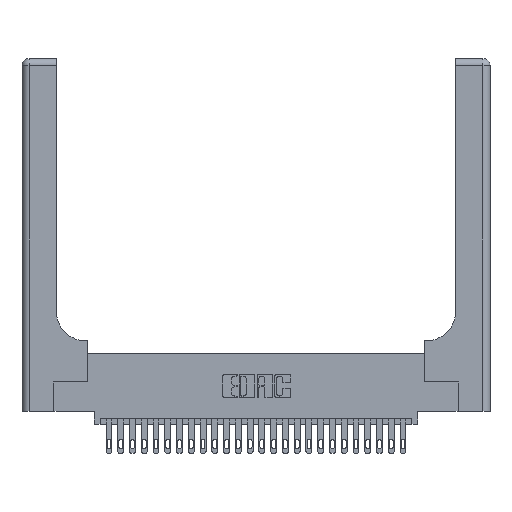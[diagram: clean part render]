
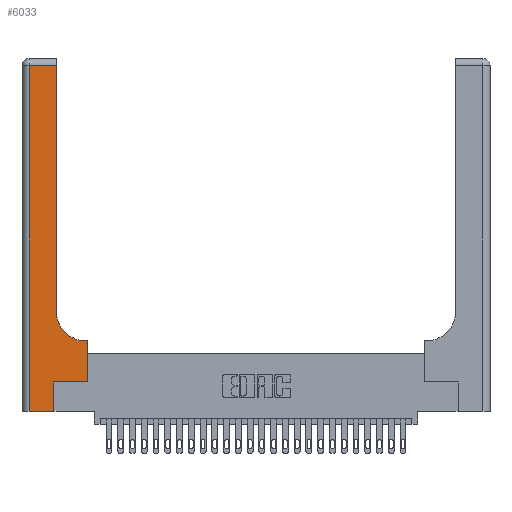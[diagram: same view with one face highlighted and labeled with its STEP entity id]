
A CAD part, top view. The second image highlights one B-rep face of the part: STEP entity #6033.
In plain terms, the highlighted planar face has unit normal (0, 0, 1).
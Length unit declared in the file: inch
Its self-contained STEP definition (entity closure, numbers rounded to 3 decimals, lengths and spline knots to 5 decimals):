
#131 = DIRECTION ( 'NONE',  ( 0., 0., -1. ) ) ;
#439 = LINE ( 'NONE', #20734, #23279 ) ;
#657 = CARTESIAN_POINT ( 'NONE',  ( 0., 2.94, 0.37 ) ) ;
#1019 = CARTESIAN_POINT ( 'NONE',  ( 0.269, 0.25, 0.37 ) ) ;
#2223 = ORIENTED_EDGE ( 'NONE', *, *, #15718, .T. ) ;
#2623 = ORIENTED_EDGE ( 'NONE', *, *, #4432, .T. ) ;
#2744 = VECTOR ( 'NONE', #12373, 39.37008 ) ;
#3171 = CARTESIAN_POINT ( 'NONE',  ( 0.269, 0.25, 0.37 ) ) ;
#3258 = VERTEX_POINT ( 'NONE', #15437 ) ;
#3762 = VERTEX_POINT ( 'NONE', #20997 ) ;
#3806 = CARTESIAN_POINT ( 'NONE',  ( 0.5585, 0.25, 0.37 ) ) ;
#3912 = VECTOR ( 'NONE', #10980, 39.37008 ) ;
#4432 = EDGE_CURVE ( 'NONE', #26588, #23386, #439, .T. ) ;
#4525 = CARTESIAN_POINT ( 'NONE',  ( 0., 3., 0.37 ) ) ;
#4573 = CARTESIAN_POINT ( 'NONE',  ( 0.2915, 0.6, 0.37 ) ) ;
#4700 = CARTESIAN_POINT ( 'NONE',  ( 0.269, 0., 0.37 ) ) ;
#5062 = VERTEX_POINT ( 'NONE', #1019 ) ;
#5669 = EDGE_CURVE ( 'NONE', #23386, #22451, #6410, .T. ) ;
#6033 = ADVANCED_FACE ( 'NONE', ( #26609 ), #24020, .F. ) ;
#6235 = CIRCLE ( 'NONE', #26925, 0.25 ) ;
#6410 = LINE ( 'NONE', #657, #2744 ) ;
#6524 = CARTESIAN_POINT ( 'NONE',  ( 0.5415, 0.85, 0.37 ) ) ;
#6826 = DIRECTION ( 'NONE',  ( 0., 1., 0. ) ) ;
#7427 = EDGE_LOOP ( 'NONE', ( #2623, #25507, #14229, #8753, #17224, #18678, #21669, #18323, #2223 ) ) ;
#8072 = EDGE_CURVE ( 'NONE', #3762, #5062, #15392, .T. ) ;
#8261 = LINE ( 'NONE', #8985, #3912 ) ;
#8492 = VERTEX_POINT ( 'NONE', #23797 ) ;
#8753 = ORIENTED_EDGE ( 'NONE', *, *, #17259, .T. ) ;
#8958 = CARTESIAN_POINT ( 'NONE',  ( 0.2915, 0.85, 0.37 ) ) ;
#8985 = CARTESIAN_POINT ( 'NONE',  ( 0.06, 3., 0.37 ) ) ;
#9343 = CARTESIAN_POINT ( 'NONE',  ( 0.2915, 2.94, 0.37 ) ) ;
#9807 = EDGE_CURVE ( 'NONE', #22451, #3258, #8261, .T. ) ;
#10113 = DIRECTION ( 'NONE',  ( 0., 1., 0. ) ) ;
#10292 = LINE ( 'NONE', #4573, #13983 ) ;
#10453 = VECTOR ( 'NONE', #11861, 39.37008 ) ;
#10499 = EDGE_CURVE ( 'NONE', #8492, #21233, #10292, .T. ) ;
#10980 = DIRECTION ( 'NONE',  ( 0., -1., 0. ) ) ;
#11861 = DIRECTION ( 'NONE',  ( 0., 1., 0. ) ) ;
#12165 = LINE ( 'NONE', #27069, #27005 ) ;
#12373 = DIRECTION ( 'NONE',  ( -1., 0., 0. ) ) ;
#12579 = VERTEX_POINT ( 'NONE', #23634 ) ;
#13983 = VECTOR ( 'NONE', #24171, 39.37008 ) ;
#14229 = ORIENTED_EDGE ( 'NONE', *, *, #9807, .T. ) ;
#14825 = LINE ( 'NONE', #3806, #10453 ) ;
#15392 = LINE ( 'NONE', #4700, #23783 ) ;
#15437 = CARTESIAN_POINT ( 'NONE',  ( 0.06, 0., 0.37 ) ) ;
#15718 = EDGE_CURVE ( 'NONE', #21233, #26588, #6235, .T. ) ;
#16834 = DIRECTION ( 'NONE',  ( 1., 0., 0. ) ) ;
#17222 = CARTESIAN_POINT ( 'NONE',  ( 0.5415, 0.6, 0.37 ) ) ;
#17224 = ORIENTED_EDGE ( 'NONE', *, *, #8072, .T. ) ;
#17259 = EDGE_CURVE ( 'NONE', #3258, #3762, #12165, .T. ) ;
#18179 = DIRECTION ( 'NONE',  ( 1., 0., 0. ) ) ;
#18323 = ORIENTED_EDGE ( 'NONE', *, *, #10499, .T. ) ;
#18451 = EDGE_CURVE ( 'NONE', #12579, #8492, #14825, .T. ) ;
#18678 = ORIENTED_EDGE ( 'NONE', *, *, #23442, .T. ) ;
#19542 = DIRECTION ( 'NONE',  ( -1., 0., 0. ) ) ;
#20734 = CARTESIAN_POINT ( 'NONE',  ( 0.2915, 3., 0.37 ) ) ;
#20775 = CARTESIAN_POINT ( 'NONE',  ( 0.06, 2.94, 0.37 ) ) ;
#20827 = VECTOR ( 'NONE', #18179, 39.37008 ) ;
#20997 = CARTESIAN_POINT ( 'NONE',  ( 0.269, 0., 0.37 ) ) ;
#21233 = VERTEX_POINT ( 'NONE', #17222 ) ;
#21669 = ORIENTED_EDGE ( 'NONE', *, *, #18451, .T. ) ;
#21988 = AXIS2_PLACEMENT_3D ( 'NONE', #4525, #24114, #19542 ) ;
#22451 = VERTEX_POINT ( 'NONE', #20775 ) ;
#22813 = LINE ( 'NONE', #3171, #20827 ) ;
#23279 = VECTOR ( 'NONE', #10113, 39.37008 ) ;
#23386 = VERTEX_POINT ( 'NONE', #9343 ) ;
#23442 = EDGE_CURVE ( 'NONE', #5062, #12579, #22813, .T. ) ;
#23634 = CARTESIAN_POINT ( 'NONE',  ( 0.5585, 0.25, 0.37 ) ) ;
#23783 = VECTOR ( 'NONE', #6826, 39.37008 ) ;
#23797 = CARTESIAN_POINT ( 'NONE',  ( 0.5585, 0.6, 0.37 ) ) ;
#24020 = PLANE ( 'NONE',  #21988 ) ;
#24114 = DIRECTION ( 'NONE',  ( 0., 0., -1. ) ) ;
#24171 = DIRECTION ( 'NONE',  ( -1., 0., 0. ) ) ;
#25507 = ORIENTED_EDGE ( 'NONE', *, *, #5669, .T. ) ;
#25887 = DIRECTION ( 'NONE',  ( 1., 0., 0. ) ) ;
#26588 = VERTEX_POINT ( 'NONE', #8958 ) ;
#26609 = FACE_OUTER_BOUND ( 'NONE', #7427, .T. ) ;
#26925 = AXIS2_PLACEMENT_3D ( 'NONE', #6524, #131, #25887 ) ;
#27005 = VECTOR ( 'NONE', #16834, 39.37008 ) ;
#27069 = CARTESIAN_POINT ( 'NONE',  ( 0., 0., 0.37 ) ) ;
